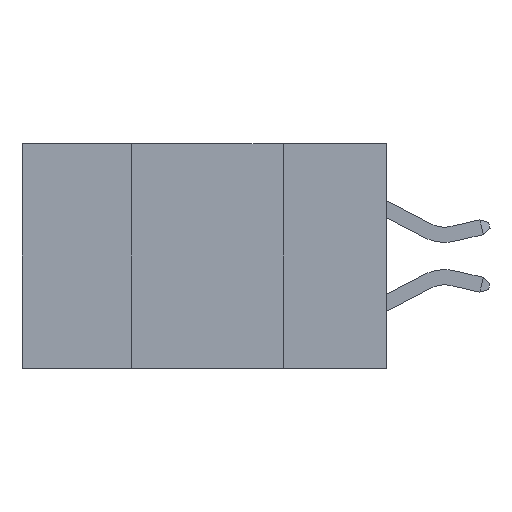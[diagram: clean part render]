
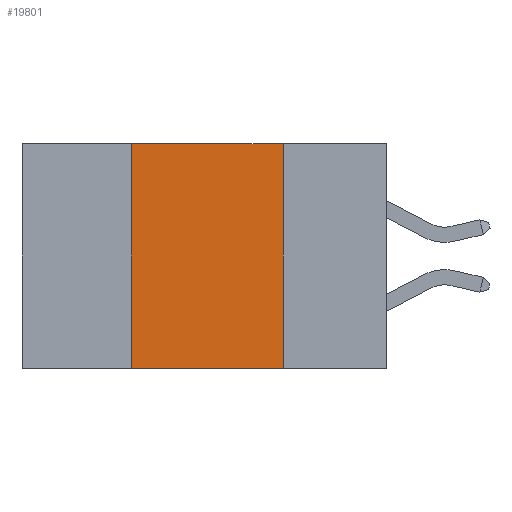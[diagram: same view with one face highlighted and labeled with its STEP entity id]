
A CAD part, left-side view. The second image highlights one B-rep face of the part: STEP entity #19801.
In plain terms, the highlighted planar face has unit normal (-1, 0, 0).
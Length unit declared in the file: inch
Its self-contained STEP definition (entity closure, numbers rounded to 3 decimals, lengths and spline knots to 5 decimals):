
#286 = CARTESIAN_POINT ( 'NONE',  ( 0., 0.17, 0. ) ) ;
#304 = PLANE ( 'NONE',  #7393 ) ;
#1781 = FACE_OUTER_BOUND ( 'NONE', #20498, .T. ) ;
#2810 = CARTESIAN_POINT ( 'NONE',  ( 0., 0.6, 0. ) ) ;
#3486 = EDGE_CURVE ( 'NONE', #19264, #13543, #5327, .T. ) ;
#3668 = DIRECTION ( 'NONE',  ( 1., 0., 0. ) ) ;
#3820 = DIRECTION ( 'NONE',  ( 0., 0., -1. ) ) ;
#4111 = ORIENTED_EDGE ( 'NONE', *, *, #16621, .T. ) ;
#4483 = DIRECTION ( 'NONE',  ( 0., -1., 0. ) ) ;
#4566 = EDGE_CURVE ( 'NONE', #20537, #6472, #5031, .T. ) ;
#5031 = LINE ( 'NONE', #13973, #14282 ) ;
#5327 = LINE ( 'NONE', #286, #13547 ) ;
#6096 = CARTESIAN_POINT ( 'NONE',  ( 0., 0.17, -0.37 ) ) ;
#6472 = VERTEX_POINT ( 'NONE', #11667 ) ;
#7393 = AXIS2_PLACEMENT_3D ( 'NONE', #13496, #3668, #15179 ) ;
#7700 = DIRECTION ( 'NONE',  ( 0., 0., 1. ) ) ;
#8529 = ORIENTED_EDGE ( 'NONE', *, *, #4566, .F. ) ;
#10318 = EDGE_CURVE ( 'NONE', #6472, #19264, #11557, .T. ) ;
#10560 = CARTESIAN_POINT ( 'NONE',  ( 0., 0.6, -0.37 ) ) ;
#11271 = ORIENTED_EDGE ( 'NONE', *, *, #10318, .F. ) ;
#11557 = LINE ( 'NONE', #2810, #19830 ) ;
#11639 = LINE ( 'NONE', #10560, #15577 ) ;
#11667 = CARTESIAN_POINT ( 'NONE',  ( 0., 0.42, 0. ) ) ;
#11925 = ORIENTED_EDGE ( 'NONE', *, *, #3486, .F. ) ;
#12234 = DIRECTION ( 'NONE',  ( 0., -1., 0. ) ) ;
#13496 = CARTESIAN_POINT ( 'NONE',  ( 0., 0.6, 0. ) ) ;
#13543 = VERTEX_POINT ( 'NONE', #6096 ) ;
#13547 = VECTOR ( 'NONE', #3820, 39.37008 ) ;
#13686 = CARTESIAN_POINT ( 'NONE',  ( 0., 0.42, -0.37 ) ) ;
#13973 = CARTESIAN_POINT ( 'NONE',  ( 0., 0.42, 0. ) ) ;
#14282 = VECTOR ( 'NONE', #7700, 39.37008 ) ;
#15179 = DIRECTION ( 'NONE',  ( 0., 0., -1. ) ) ;
#15577 = VECTOR ( 'NONE', #12234, 39.37008 ) ;
#16621 = EDGE_CURVE ( 'NONE', #20537, #13543, #11639, .T. ) ;
#19264 = VERTEX_POINT ( 'NONE', #20469 ) ;
#19801 = ADVANCED_FACE ( 'NONE', ( #1781 ), #304, .F. ) ;
#19830 = VECTOR ( 'NONE', #4483, 39.37008 ) ;
#20469 = CARTESIAN_POINT ( 'NONE',  ( 0., 0.17, 0. ) ) ;
#20498 = EDGE_LOOP ( 'NONE', ( #11925, #11271, #8529, #4111 ) ) ;
#20537 = VERTEX_POINT ( 'NONE', #13686 ) ;
